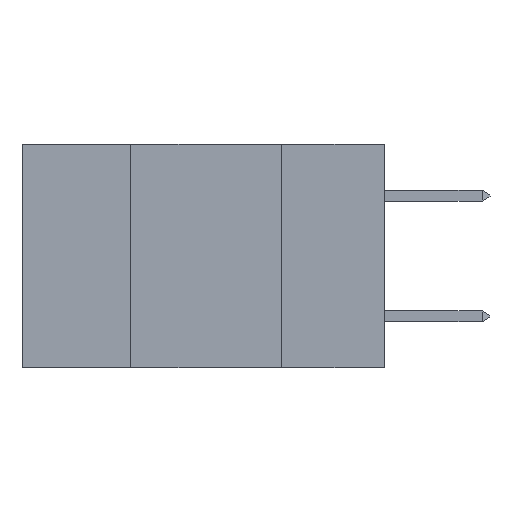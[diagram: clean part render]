
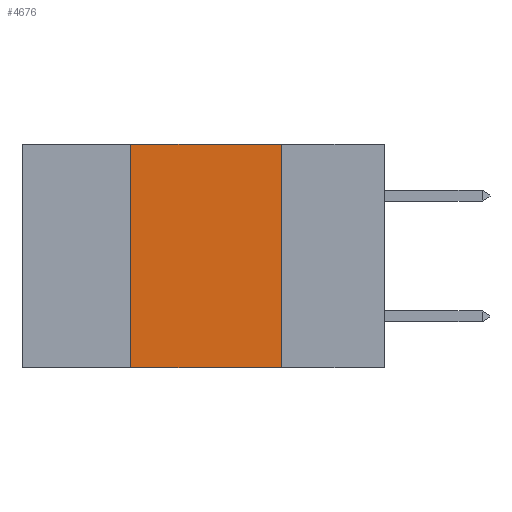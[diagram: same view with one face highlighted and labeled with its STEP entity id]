
A CAD part, left-side view. The second image highlights one B-rep face of the part: STEP entity #4676.
In plain terms, the highlighted planar face has unit normal (-1, 0, 0).
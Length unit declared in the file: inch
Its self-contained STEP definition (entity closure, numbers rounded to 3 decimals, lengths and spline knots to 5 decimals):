
#294 = ORIENTED_EDGE ( 'NONE', *, *, #3175, .F. ) ;
#327 = VERTEX_POINT ( 'NONE', #10065 ) ;
#878 = VERTEX_POINT ( 'NONE', #4322 ) ;
#1110 = CARTESIAN_POINT ( 'NONE',  ( 0., 0.17, 0. ) ) ;
#1914 = CARTESIAN_POINT ( 'NONE',  ( 0., 0.42, 0. ) ) ;
#2181 = CARTESIAN_POINT ( 'NONE',  ( 0., 0.6, 0. ) ) ;
#2341 = DIRECTION ( 'NONE',  ( 0., 0., -1. ) ) ;
#2382 = VECTOR ( 'NONE', #4530, 39.37008 ) ;
#3175 = EDGE_CURVE ( 'NONE', #14102, #13932, #4275, .T. ) ;
#3836 = LINE ( 'NONE', #8386, #8621 ) ;
#4275 = LINE ( 'NONE', #2181, #13883 ) ;
#4322 = CARTESIAN_POINT ( 'NONE',  ( 0., 0.17, -0.37 ) ) ;
#4530 = DIRECTION ( 'NONE',  ( 0., -1., 0. ) ) ;
#4605 = CARTESIAN_POINT ( 'NONE',  ( 0., 0.6, -0.37 ) ) ;
#4676 = ADVANCED_FACE ( 'NONE', ( #12121 ), #9847, .F. ) ;
#6107 = EDGE_LOOP ( 'NONE', ( #8191, #294, #6827, #13741 ) ) ;
#6827 = ORIENTED_EDGE ( 'NONE', *, *, #14598, .F. ) ;
#8191 = ORIENTED_EDGE ( 'NONE', *, *, #10757, .F. ) ;
#8386 = CARTESIAN_POINT ( 'NONE',  ( 0., 0.17, 0. ) ) ;
#8621 = VECTOR ( 'NONE', #2341, 39.37008 ) ;
#8664 = CARTESIAN_POINT ( 'NONE',  ( 0., 0.6, 0. ) ) ;
#8805 = DIRECTION ( 'NONE',  ( 0., 0., -1. ) ) ;
#8851 = EDGE_CURVE ( 'NONE', #327, #878, #10188, .T. ) ;
#9847 = PLANE ( 'NONE',  #10157 ) ;
#10065 = CARTESIAN_POINT ( 'NONE',  ( 0., 0.42, -0.37 ) ) ;
#10157 = AXIS2_PLACEMENT_3D ( 'NONE', #8664, #14497, #8805 ) ;
#10188 = LINE ( 'NONE', #4605, #2382 ) ;
#10334 = VECTOR ( 'NONE', #12093, 39.37008 ) ;
#10757 = EDGE_CURVE ( 'NONE', #13932, #878, #3836, .T. ) ;
#12093 = DIRECTION ( 'NONE',  ( 0., 0., 1. ) ) ;
#12112 = CARTESIAN_POINT ( 'NONE',  ( 0., 0.42, 0. ) ) ;
#12121 = FACE_OUTER_BOUND ( 'NONE', #6107, .T. ) ;
#12421 = DIRECTION ( 'NONE',  ( 0., -1., 0. ) ) ;
#13741 = ORIENTED_EDGE ( 'NONE', *, *, #8851, .T. ) ;
#13883 = VECTOR ( 'NONE', #12421, 39.37008 ) ;
#13932 = VERTEX_POINT ( 'NONE', #1110 ) ;
#14102 = VERTEX_POINT ( 'NONE', #12112 ) ;
#14334 = LINE ( 'NONE', #1914, #10334 ) ;
#14497 = DIRECTION ( 'NONE',  ( 1., 0., 0. ) ) ;
#14598 = EDGE_CURVE ( 'NONE', #327, #14102, #14334, .T. ) ;
